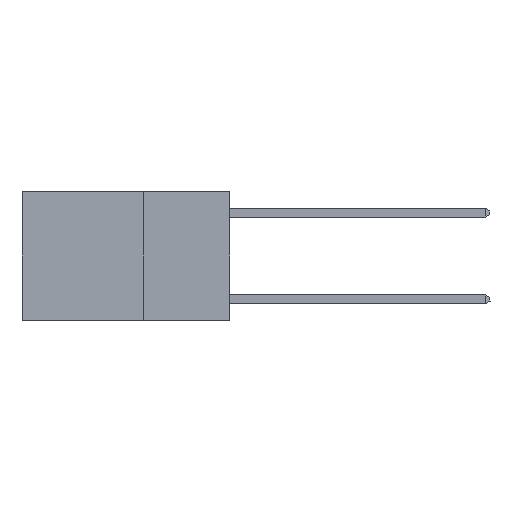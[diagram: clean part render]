
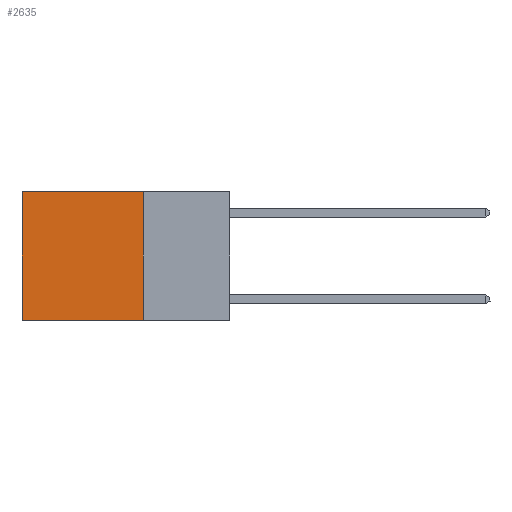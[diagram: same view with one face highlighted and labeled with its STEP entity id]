
A CAD part, left-side view. The second image highlights one B-rep face of the part: STEP entity #2635.
In plain terms, the highlighted planar face has unit normal (-1, 0, 0).
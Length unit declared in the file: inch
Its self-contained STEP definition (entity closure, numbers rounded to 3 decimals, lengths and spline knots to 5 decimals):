
#241 = VECTOR ( 'NONE', #9559, 39.37008 ) ;
#1253 = EDGE_CURVE ( 'NONE', #9375, #11670, #11625, .T. ) ;
#1481 = EDGE_CURVE ( 'NONE', #7479, #9375, #6606, .T. ) ;
#1556 = DIRECTION ( 'NONE',  ( 1., 0., 0. ) ) ;
#2371 = DIRECTION ( 'NONE',  ( 0., 1., 0. ) ) ;
#2425 = EDGE_CURVE ( 'NONE', #7423, #11670, #7579, .T. ) ;
#2507 = AXIS2_PLACEMENT_3D ( 'NONE', #9852, #1556, #4378 ) ;
#2635 = ADVANCED_FACE ( 'NONE', ( #11876 ), #10656, .F. ) ;
#3183 = CARTESIAN_POINT ( 'NONE',  ( 0.2625, 0.6, 0. ) ) ;
#4003 = VECTOR ( 'NONE', #2371, 39.37008 ) ;
#4378 = DIRECTION ( 'NONE',  ( 0., 0., -1. ) ) ;
#4625 = CARTESIAN_POINT ( 'NONE',  ( 0.2625, 0.25, -0.37 ) ) ;
#4800 = CARTESIAN_POINT ( 'NONE',  ( 0.2625, 0.25, 0. ) ) ;
#4979 = CARTESIAN_POINT ( 'NONE',  ( 0.2625, 0.6, -0.37 ) ) ;
#5575 = ORIENTED_EDGE ( 'NONE', *, *, #1253, .T. ) ;
#6047 = DIRECTION ( 'NONE',  ( 0., 0., -1. ) ) ;
#6350 = VECTOR ( 'NONE', #6047, 39.37008 ) ;
#6606 = LINE ( 'NONE', #8834, #8192 ) ;
#7423 = VERTEX_POINT ( 'NONE', #10339 ) ;
#7479 = VERTEX_POINT ( 'NONE', #4800 ) ;
#7553 = EDGE_CURVE ( 'NONE', #7479, #7423, #9156, .T. ) ;
#7579 = LINE ( 'NONE', #4625, #4003 ) ;
#8153 = EDGE_LOOP ( 'NONE', ( #5575, #11061, #9569, #10945 ) ) ;
#8192 = VECTOR ( 'NONE', #11563, 39.37008 ) ;
#8435 = CARTESIAN_POINT ( 'NONE',  ( 0.2625, 0.6, 0. ) ) ;
#8834 = CARTESIAN_POINT ( 'NONE',  ( 0.2625, 0.25, 0. ) ) ;
#9156 = LINE ( 'NONE', #11498, #241 ) ;
#9375 = VERTEX_POINT ( 'NONE', #8435 ) ;
#9559 = DIRECTION ( 'NONE',  ( 0., 0., -1. ) ) ;
#9569 = ORIENTED_EDGE ( 'NONE', *, *, #7553, .F. ) ;
#9852 = CARTESIAN_POINT ( 'NONE',  ( 0.2625, 0.25, 0. ) ) ;
#10339 = CARTESIAN_POINT ( 'NONE',  ( 0.2625, 0.25, -0.37 ) ) ;
#10656 = PLANE ( 'NONE',  #2507 ) ;
#10945 = ORIENTED_EDGE ( 'NONE', *, *, #1481, .T. ) ;
#11061 = ORIENTED_EDGE ( 'NONE', *, *, #2425, .F. ) ;
#11498 = CARTESIAN_POINT ( 'NONE',  ( 0.2625, 0.25, 0. ) ) ;
#11563 = DIRECTION ( 'NONE',  ( 0., 1., 0. ) ) ;
#11625 = LINE ( 'NONE', #3183, #6350 ) ;
#11670 = VERTEX_POINT ( 'NONE', #4979 ) ;
#11876 = FACE_OUTER_BOUND ( 'NONE', #8153, .T. ) ;
